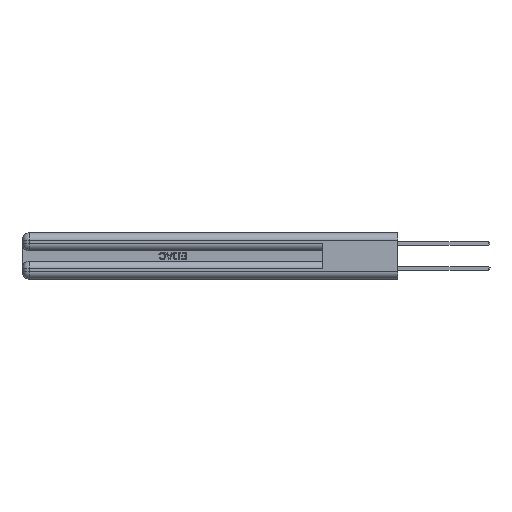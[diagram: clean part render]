
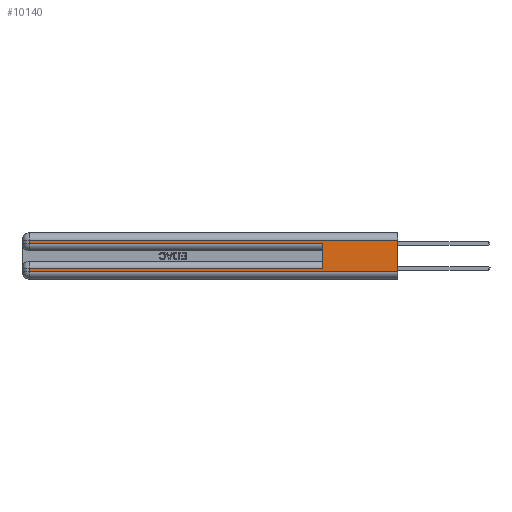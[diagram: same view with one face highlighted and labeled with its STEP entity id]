
A CAD part, left-side view. The second image highlights one B-rep face of the part: STEP entity #10140.
In plain terms, the highlighted planar face has unit normal (-1, 0, 0).
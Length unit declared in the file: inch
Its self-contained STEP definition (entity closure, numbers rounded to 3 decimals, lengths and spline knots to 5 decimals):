
#670 = VECTOR ( 'NONE', #24250, 39.37008 ) ;
#1167 = VERTEX_POINT ( 'NONE', #14603 ) ;
#1223 = LINE ( 'NONE', #31688, #34093 ) ;
#1241 = EDGE_LOOP ( 'NONE', ( #33895, #23509, #12387, #24545, #25800, #37819, #33836, #3913 ) ) ;
#1648 = CARTESIAN_POINT ( 'NONE',  ( 0., 0., 0.31 ) ) ;
#2607 = CARTESIAN_POINT ( 'NONE',  ( 0., 0., 0.37 ) ) ;
#2755 = PLANE ( 'NONE',  #44069 ) ;
#3913 = ORIENTED_EDGE ( 'NONE', *, *, #29922, .T. ) ;
#4245 = VECTOR ( 'NONE', #23124, 39.37008 ) ;
#6261 = CARTESIAN_POINT ( 'NONE',  ( 0., 0., 0.285 ) ) ;
#7613 = EDGE_CURVE ( 'NONE', #35310, #25018, #33580, .T. ) ;
#7695 = EDGE_CURVE ( 'NONE', #25018, #28313, #21212, .T. ) ;
#9988 = DIRECTION ( 'NONE',  ( 0., 0., -1. ) ) ;
#10132 = EDGE_CURVE ( 'NONE', #35310, #18124, #19897, .T. ) ;
#10140 = ADVANCED_FACE ( 'NONE', ( #21069 ), #2755, .F. ) ;
#10159 = DIRECTION ( 'NONE',  ( 1., 0., 0. ) ) ;
#12231 = DIRECTION ( 'NONE',  ( 0., 1., 0. ) ) ;
#12387 = ORIENTED_EDGE ( 'NONE', *, *, #7695, .T. ) ;
#12867 = DIRECTION ( 'NONE',  ( 0., -1., 0. ) ) ;
#12909 = VECTOR ( 'NONE', #12867, 39.37008 ) ;
#14273 = VERTEX_POINT ( 'NONE', #45363 ) ;
#14603 = CARTESIAN_POINT ( 'NONE',  ( 0., 0.6, 0.285 ) ) ;
#15252 = LINE ( 'NONE', #35005, #44003 ) ;
#16976 = VERTEX_POINT ( 'NONE', #45880 ) ;
#17652 = EDGE_CURVE ( 'NONE', #14273, #48351, #15252, .T. ) ;
#17696 = CARTESIAN_POINT ( 'NONE',  ( 0., 0., 0.37 ) ) ;
#18124 = VERTEX_POINT ( 'NONE', #45601 ) ;
#19756 = CARTESIAN_POINT ( 'NONE',  ( 0., 2.94, 0.31 ) ) ;
#19897 = LINE ( 'NONE', #2607, #42793 ) ;
#20217 = DIRECTION ( 'NONE',  ( 0., 0., -1. ) ) ;
#20635 = VECTOR ( 'NONE', #21345, 39.37008 ) ;
#21069 = FACE_OUTER_BOUND ( 'NONE', #1241, .T. ) ;
#21212 = LINE ( 'NONE', #42782, #670 ) ;
#21345 = DIRECTION ( 'NONE',  ( 0., -1., 0. ) ) ;
#22856 = LINE ( 'NONE', #41710, #12909 ) ;
#23124 = DIRECTION ( 'NONE',  ( 0., 1., 0. ) ) ;
#23509 = ORIENTED_EDGE ( 'NONE', *, *, #7613, .T. ) ;
#24117 = EDGE_CURVE ( 'NONE', #48351, #16976, #1223, .T. ) ;
#24250 = DIRECTION ( 'NONE',  ( 0., 0., -1. ) ) ;
#24545 = ORIENTED_EDGE ( 'NONE', *, *, #28469, .T. ) ;
#25018 = VERTEX_POINT ( 'NONE', #19756 ) ;
#25245 = CARTESIAN_POINT ( 'NONE',  ( 0., 0.6, 0.145 ) ) ;
#25800 = ORIENTED_EDGE ( 'NONE', *, *, #27770, .F. ) ;
#27770 = EDGE_CURVE ( 'NONE', #14273, #1167, #47748, .T. ) ;
#28313 = VERTEX_POINT ( 'NONE', #35471 ) ;
#28469 = EDGE_CURVE ( 'NONE', #28313, #1167, #30608, .T. ) ;
#29650 = DIRECTION ( 'NONE',  ( 0., 0., 1. ) ) ;
#29922 = EDGE_CURVE ( 'NONE', #16976, #18124, #22856, .T. ) ;
#30204 = CARTESIAN_POINT ( 'NONE',  ( 0., 2.94, 0.085 ) ) ;
#30608 = LINE ( 'NONE', #6261, #20635 ) ;
#31688 = CARTESIAN_POINT ( 'NONE',  ( 0., 2.94, 0.37 ) ) ;
#32758 = DIRECTION ( 'NONE',  ( 0., 0., -1. ) ) ;
#33580 = LINE ( 'NONE', #41986, #4245 ) ;
#33836 = ORIENTED_EDGE ( 'NONE', *, *, #24117, .T. ) ;
#33895 = ORIENTED_EDGE ( 'NONE', *, *, #10132, .F. ) ;
#34093 = VECTOR ( 'NONE', #20217, 39.37008 ) ;
#35005 = CARTESIAN_POINT ( 'NONE',  ( 0., 0., 0.085 ) ) ;
#35310 = VERTEX_POINT ( 'NONE', #1648 ) ;
#35471 = CARTESIAN_POINT ( 'NONE',  ( 0., 2.94, 0.285 ) ) ;
#36577 = VECTOR ( 'NONE', #29650, 39.37008 ) ;
#37819 = ORIENTED_EDGE ( 'NONE', *, *, #17652, .T. ) ;
#41710 = CARTESIAN_POINT ( 'NONE',  ( 0., 0., 0.06 ) ) ;
#41986 = CARTESIAN_POINT ( 'NONE',  ( 0., 0., 0.31 ) ) ;
#42782 = CARTESIAN_POINT ( 'NONE',  ( 0., 2.94, 0.37 ) ) ;
#42793 = VECTOR ( 'NONE', #9988, 39.37008 ) ;
#44003 = VECTOR ( 'NONE', #12231, 39.37008 ) ;
#44069 = AXIS2_PLACEMENT_3D ( 'NONE', #17696, #10159, #32758 ) ;
#45363 = CARTESIAN_POINT ( 'NONE',  ( 0., 0.6, 0.085 ) ) ;
#45601 = CARTESIAN_POINT ( 'NONE',  ( 0., 0., 0.06 ) ) ;
#45880 = CARTESIAN_POINT ( 'NONE',  ( 0., 2.94, 0.06 ) ) ;
#47748 = LINE ( 'NONE', #25245, #36577 ) ;
#48351 = VERTEX_POINT ( 'NONE', #30204 ) ;
